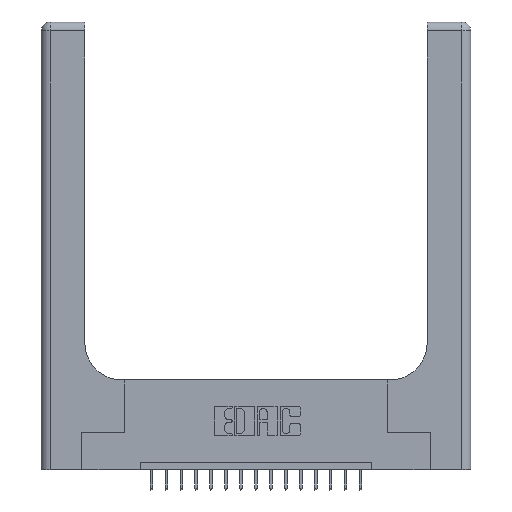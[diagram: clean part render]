
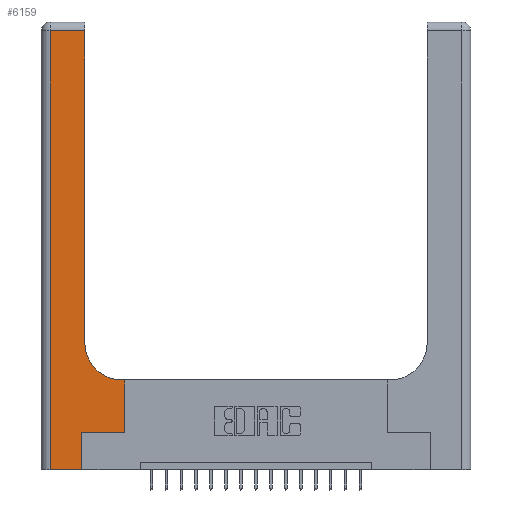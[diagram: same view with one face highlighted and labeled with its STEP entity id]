
A CAD part, top view. The second image highlights one B-rep face of the part: STEP entity #6159.
In plain terms, the highlighted planar face has unit normal (0, 0, 1).
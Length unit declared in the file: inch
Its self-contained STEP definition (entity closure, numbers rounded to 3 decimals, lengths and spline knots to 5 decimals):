
#118 = ORIENTED_EDGE ( 'NONE', *, *, #18437, .T. ) ;
#194 = EDGE_CURVE ( 'NONE', #2182, #19820, #15070, .T. ) ;
#386 = VECTOR ( 'NONE', #18818, 39.37008 ) ;
#543 = EDGE_CURVE ( 'NONE', #12325, #6580, #12433, .T. ) ;
#588 = ORIENTED_EDGE ( 'NONE', *, *, #194, .T. ) ;
#1043 = VECTOR ( 'NONE', #17872, 39.37008 ) ;
#1050 = DIRECTION ( 'NONE',  ( 0., 1., 0. ) ) ;
#1295 = VERTEX_POINT ( 'NONE', #3975 ) ;
#1511 = CARTESIAN_POINT ( 'NONE',  ( 0.2915, 3., 0.37 ) ) ;
#1745 = LINE ( 'NONE', #14092, #2044 ) ;
#1927 = EDGE_CURVE ( 'NONE', #17529, #3201, #12894, .T. ) ;
#1987 = CARTESIAN_POINT ( 'NONE',  ( 0.06, 2.94, 0.37 ) ) ;
#2041 = CARTESIAN_POINT ( 'NONE',  ( 0., 2.94, 0.37 ) ) ;
#2044 = VECTOR ( 'NONE', #14404, 39.37008 ) ;
#2182 = VERTEX_POINT ( 'NONE', #2237 ) ;
#2237 = CARTESIAN_POINT ( 'NONE',  ( 0.5585, 0.25, 0.37 ) ) ;
#2389 = CARTESIAN_POINT ( 'NONE',  ( 0.5585, 0.6, 0.37 ) ) ;
#2809 = CARTESIAN_POINT ( 'NONE',  ( 0., 0., 0.37 ) ) ;
#3201 = VERTEX_POINT ( 'NONE', #8326 ) ;
#3241 = DIRECTION ( 'NONE',  ( -1., 0., 0. ) ) ;
#3270 = CARTESIAN_POINT ( 'NONE',  ( 0.269, 0.25, 0.37 ) ) ;
#3833 = ORIENTED_EDGE ( 'NONE', *, *, #1927, .T. ) ;
#3975 = CARTESIAN_POINT ( 'NONE',  ( 0.269, 0., 0.37 ) ) ;
#4011 = VERTEX_POINT ( 'NONE', #14195 ) ;
#4017 = CARTESIAN_POINT ( 'NONE',  ( 0.2915, 2.94, 0.37 ) ) ;
#4156 = EDGE_CURVE ( 'NONE', #6580, #17529, #14710, .T. ) ;
#4333 = LINE ( 'NONE', #2809, #14548 ) ;
#4724 = DIRECTION ( 'NONE',  ( -1., 0., 0. ) ) ;
#4824 = EDGE_CURVE ( 'NONE', #4878, #12325, #9267, .T. ) ;
#4878 = VERTEX_POINT ( 'NONE', #15044 ) ;
#5834 = VECTOR ( 'NONE', #6524, 39.37008 ) ;
#6159 = ADVANCED_FACE ( 'NONE', ( #12503 ), #14039, .F. ) ;
#6524 = DIRECTION ( 'NONE',  ( 1., 0., 0. ) ) ;
#6580 = VERTEX_POINT ( 'NONE', #4017 ) ;
#7056 = DIRECTION ( 'NONE',  ( 1., 0., 0. ) ) ;
#7068 = EDGE_CURVE ( 'NONE', #3201, #1295, #4333, .T. ) ;
#8169 = LINE ( 'NONE', #3270, #5834 ) ;
#8326 = CARTESIAN_POINT ( 'NONE',  ( 0.06, 0., 0.37 ) ) ;
#9267 = CIRCLE ( 'NONE', #14820, 0.25 ) ;
#9297 = AXIS2_PLACEMENT_3D ( 'NONE', #18737, #15596, #4724 ) ;
#9459 = EDGE_LOOP ( 'NONE', ( #12877, #12466, #3833, #17764, #118, #9934, #588, #14366, #17112 ) ) ;
#9749 = CARTESIAN_POINT ( 'NONE',  ( 0.06, 3., 0.37 ) ) ;
#9934 = ORIENTED_EDGE ( 'NONE', *, *, #11022, .T. ) ;
#10163 = VECTOR ( 'NONE', #1050, 39.37008 ) ;
#10789 = VECTOR ( 'NONE', #20176, 39.37008 ) ;
#10795 = CARTESIAN_POINT ( 'NONE',  ( 0.2915, 0.85, 0.37 ) ) ;
#11022 = EDGE_CURVE ( 'NONE', #4011, #2182, #8169, .T. ) ;
#11027 = LINE ( 'NONE', #17271, #19287 ) ;
#11770 = DIRECTION ( 'NONE',  ( 0., 0., -1. ) ) ;
#12325 = VERTEX_POINT ( 'NONE', #10795 ) ;
#12433 = LINE ( 'NONE', #1511, #10789 ) ;
#12466 = ORIENTED_EDGE ( 'NONE', *, *, #4156, .T. ) ;
#12503 = FACE_OUTER_BOUND ( 'NONE', #9459, .T. ) ;
#12877 = ORIENTED_EDGE ( 'NONE', *, *, #543, .T. ) ;
#12894 = LINE ( 'NONE', #9749, #386 ) ;
#14039 = PLANE ( 'NONE',  #9297 ) ;
#14092 = CARTESIAN_POINT ( 'NONE',  ( 0.269, 0., 0.37 ) ) ;
#14195 = CARTESIAN_POINT ( 'NONE',  ( 0.269, 0.25, 0.37 ) ) ;
#14366 = ORIENTED_EDGE ( 'NONE', *, *, #14943, .T. ) ;
#14404 = DIRECTION ( 'NONE',  ( 0., 1., 0. ) ) ;
#14548 = VECTOR ( 'NONE', #17781, 39.37008 ) ;
#14710 = LINE ( 'NONE', #2041, #1043 ) ;
#14820 = AXIS2_PLACEMENT_3D ( 'NONE', #19900, #11770, #7056 ) ;
#14943 = EDGE_CURVE ( 'NONE', #19820, #4878, #11027, .T. ) ;
#15044 = CARTESIAN_POINT ( 'NONE',  ( 0.5415, 0.6, 0.37 ) ) ;
#15070 = LINE ( 'NONE', #16517, #10163 ) ;
#15596 = DIRECTION ( 'NONE',  ( 0., 0., -1. ) ) ;
#16517 = CARTESIAN_POINT ( 'NONE',  ( 0.5585, 0.25, 0.37 ) ) ;
#17112 = ORIENTED_EDGE ( 'NONE', *, *, #4824, .T. ) ;
#17271 = CARTESIAN_POINT ( 'NONE',  ( 0.2915, 0.6, 0.37 ) ) ;
#17529 = VERTEX_POINT ( 'NONE', #1987 ) ;
#17764 = ORIENTED_EDGE ( 'NONE', *, *, #7068, .T. ) ;
#17781 = DIRECTION ( 'NONE',  ( 1., 0., 0. ) ) ;
#17872 = DIRECTION ( 'NONE',  ( -1., 0., 0. ) ) ;
#18437 = EDGE_CURVE ( 'NONE', #1295, #4011, #1745, .T. ) ;
#18737 = CARTESIAN_POINT ( 'NONE',  ( 0., 3., 0.37 ) ) ;
#18818 = DIRECTION ( 'NONE',  ( 0., -1., 0. ) ) ;
#19287 = VECTOR ( 'NONE', #3241, 39.37008 ) ;
#19820 = VERTEX_POINT ( 'NONE', #2389 ) ;
#19900 = CARTESIAN_POINT ( 'NONE',  ( 0.5415, 0.85, 0.37 ) ) ;
#20176 = DIRECTION ( 'NONE',  ( 0., 1., 0. ) ) ;
